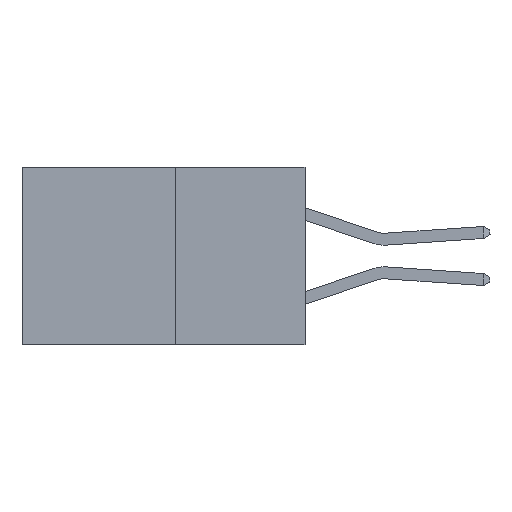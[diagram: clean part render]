
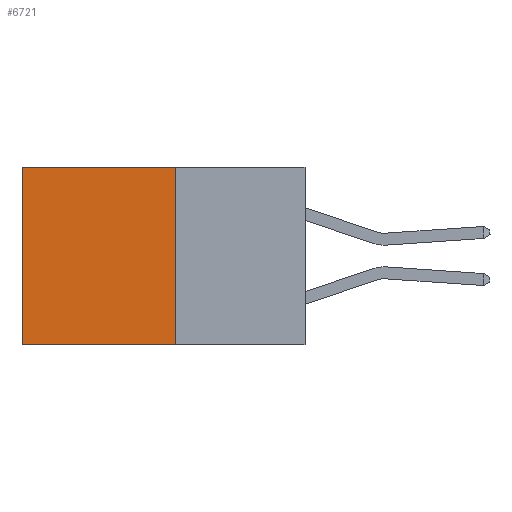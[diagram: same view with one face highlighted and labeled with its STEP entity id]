
A CAD part, left-side view. The second image highlights one B-rep face of the part: STEP entity #6721.
In plain terms, the highlighted planar face has unit normal (-1, 0, 0).
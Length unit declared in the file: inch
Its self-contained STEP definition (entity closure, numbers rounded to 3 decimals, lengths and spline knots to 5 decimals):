
#877 = DIRECTION ( 'NONE',  ( 1., 0., 0. ) ) ;
#1004 = LINE ( 'NONE', #10507, #12812 ) ;
#1139 = CARTESIAN_POINT ( 'NONE',  ( 0.277, 0.27, 0. ) ) ;
#1660 = EDGE_CURVE ( 'NONE', #12302, #13273, #1824, .T. ) ;
#1824 = LINE ( 'NONE', #11958, #13590 ) ;
#2349 = VECTOR ( 'NONE', #4120, 39.37008 ) ;
#3105 = VERTEX_POINT ( 'NONE', #1139 ) ;
#4039 = DIRECTION ( 'NONE',  ( 0., 0., -1. ) ) ;
#4120 = DIRECTION ( 'NONE',  ( 0., 1., 0. ) ) ;
#4936 = CARTESIAN_POINT ( 'NONE',  ( 0.277, 0.59, -0.37 ) ) ;
#5262 = FACE_OUTER_BOUND ( 'NONE', #7211, .T. ) ;
#5653 = ORIENTED_EDGE ( 'NONE', *, *, #9546, .F. ) ;
#5678 = DIRECTION ( 'NONE',  ( 0., 0., -1. ) ) ;
#5956 = DIRECTION ( 'NONE',  ( 0., 1., 0. ) ) ;
#6197 = AXIS2_PLACEMENT_3D ( 'NONE', #11210, #877, #8966 ) ;
#6375 = LINE ( 'NONE', #11349, #12384 ) ;
#6415 = CARTESIAN_POINT ( 'NONE',  ( 0.277, 0.27, -0.37 ) ) ;
#6713 = CARTESIAN_POINT ( 'NONE',  ( 0.277, 0.59, 0. ) ) ;
#6721 = ADVANCED_FACE ( 'NONE', ( #5262 ), #14603, .F. ) ;
#7211 = EDGE_LOOP ( 'NONE', ( #12597, #5653, #11011, #11252 ) ) ;
#8966 = DIRECTION ( 'NONE',  ( 0., 0., -1. ) ) ;
#9213 = EDGE_CURVE ( 'NONE', #3105, #12302, #1004, .T. ) ;
#9546 = EDGE_CURVE ( 'NONE', #9651, #13273, #14464, .T. ) ;
#9651 = VERTEX_POINT ( 'NONE', #14519 ) ;
#10507 = CARTESIAN_POINT ( 'NONE',  ( 0.277, 0.27, 0. ) ) ;
#11011 = ORIENTED_EDGE ( 'NONE', *, *, #13026, .F. ) ;
#11210 = CARTESIAN_POINT ( 'NONE',  ( 0.277, 0.27, -0.37 ) ) ;
#11252 = ORIENTED_EDGE ( 'NONE', *, *, #9213, .T. ) ;
#11349 = CARTESIAN_POINT ( 'NONE',  ( 0.277, 0.27, -0.37 ) ) ;
#11958 = CARTESIAN_POINT ( 'NONE',  ( 0.277, 0.59, -0.37 ) ) ;
#12302 = VERTEX_POINT ( 'NONE', #6713 ) ;
#12384 = VECTOR ( 'NONE', #5678, 39.37008 ) ;
#12597 = ORIENTED_EDGE ( 'NONE', *, *, #1660, .T. ) ;
#12812 = VECTOR ( 'NONE', #5956, 39.37008 ) ;
#13026 = EDGE_CURVE ( 'NONE', #3105, #9651, #6375, .T. ) ;
#13273 = VERTEX_POINT ( 'NONE', #4936 ) ;
#13590 = VECTOR ( 'NONE', #4039, 39.37008 ) ;
#14464 = LINE ( 'NONE', #6415, #2349 ) ;
#14519 = CARTESIAN_POINT ( 'NONE',  ( 0.277, 0.27, -0.37 ) ) ;
#14603 = PLANE ( 'NONE',  #6197 ) ;
